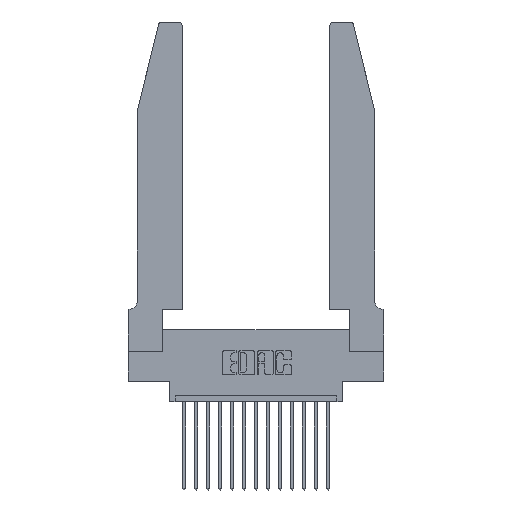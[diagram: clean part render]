
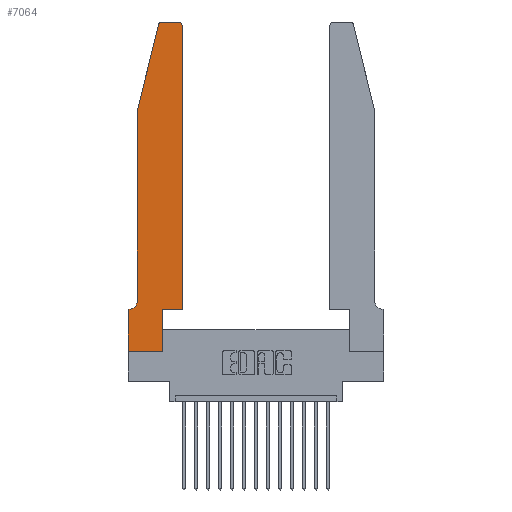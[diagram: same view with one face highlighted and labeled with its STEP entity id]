
A CAD part, top view. The second image highlights one B-rep face of the part: STEP entity #7064.
In plain terms, the highlighted planar face has unit normal (0, 0, 1).
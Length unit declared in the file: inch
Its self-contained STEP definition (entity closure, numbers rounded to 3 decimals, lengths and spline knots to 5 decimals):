
#534 = CARTESIAN_POINT ( 'NONE',  ( 0.2605, 2.75, 0.37 ) ) ;
#580 = ORIENTED_EDGE ( 'NONE', *, *, #16881, .T. ) ;
#1202 = FACE_OUTER_BOUND ( 'NONE', #14484, .T. ) ;
#1241 = VERTEX_POINT ( 'NONE', #10068 ) ;
#1324 = DIRECTION ( 'NONE',  ( 0., -1., 0. ) ) ;
#1689 = VECTOR ( 'NONE', #11862, 39.37008 ) ;
#1705 = LINE ( 'NONE', #17944, #4839 ) ;
#1820 = CARTESIAN_POINT ( 'NONE',  ( 0.0755, 0.42, 0.37 ) ) ;
#1891 = PLANE ( 'NONE',  #5517 ) ;
#2153 = CARTESIAN_POINT ( 'NONE',  ( 0.2865, 0.35, 0.37 ) ) ;
#2384 = ORIENTED_EDGE ( 'NONE', *, *, #9184, .T. ) ;
#2760 = DIRECTION ( 'NONE',  ( -0.239, -0.971, 0. ) ) ;
#2847 = ORIENTED_EDGE ( 'NONE', *, *, #17424, .T. ) ;
#3040 = LINE ( 'NONE', #8576, #8632 ) ;
#3177 = CARTESIAN_POINT ( 'NONE',  ( 0.284, 2.75, 0.37 ) ) ;
#3264 = ORIENTED_EDGE ( 'NONE', *, *, #9776, .T. ) ;
#3312 = DIRECTION ( 'NONE',  ( 0., 0., -1. ) ) ;
#3365 = VERTEX_POINT ( 'NONE', #1820 ) ;
#3503 = EDGE_CURVE ( 'NONE', #1241, #18596, #6241, .T. ) ;
#3515 = CIRCLE ( 'NONE', #6505, 0.03 ) ;
#3594 = CARTESIAN_POINT ( 'NONE',  ( 0.0755, 2., 0.37 ) ) ;
#3656 = LINE ( 'NONE', #2153, #18417 ) ;
#3830 = ORIENTED_EDGE ( 'NONE', *, *, #5843, .T. ) ;
#3967 = CARTESIAN_POINT ( 'NONE',  ( 0.4505, 0.35, 0.37 ) ) ;
#4839 = VECTOR ( 'NONE', #15191, 39.37008 ) ;
#5005 = ORIENTED_EDGE ( 'NONE', *, *, #8663, .T. ) ;
#5063 = CARTESIAN_POINT ( 'NONE',  ( 0.284, 2.72, 0.37 ) ) ;
#5140 = LINE ( 'NONE', #12147, #12791 ) ;
#5157 = CARTESIAN_POINT ( 'NONE',  ( 0.4505, 0.35, 0.37 ) ) ;
#5517 = AXIS2_PLACEMENT_3D ( 'NONE', #14723, #13571, #9292 ) ;
#5765 = CARTESIAN_POINT ( 'NONE',  ( 0.4205, 2.75, 0.37 ) ) ;
#5801 = ORIENTED_EDGE ( 'NONE', *, *, #14795, .T. ) ;
#5843 = EDGE_CURVE ( 'NONE', #7129, #14209, #3040, .T. ) ;
#5889 = AXIS2_PLACEMENT_3D ( 'NONE', #5063, #15081, #16521 ) ;
#6227 = VECTOR ( 'NONE', #12973, 39.37008 ) ;
#6241 = LINE ( 'NONE', #3967, #13441 ) ;
#6505 = AXIS2_PLACEMENT_3D ( 'NONE', #15580, #8442, #18453 ) ;
#6747 = CARTESIAN_POINT ( 'NONE',  ( 0.25487, 2.72718, 0.37 ) ) ;
#7064 = ADVANCED_FACE ( 'NONE', ( #1202 ), #1891, .T. ) ;
#7129 = VERTEX_POINT ( 'NONE', #6747 ) ;
#7432 = VERTEX_POINT ( 'NONE', #5765 ) ;
#7665 = VERTEX_POINT ( 'NONE', #8841 ) ;
#7791 = DIRECTION ( 'NONE',  ( 0., 1., 0. ) ) ;
#7884 = VECTOR ( 'NONE', #1324, 39.37008 ) ;
#8008 = VERTEX_POINT ( 'NONE', #9509 ) ;
#8344 = CARTESIAN_POINT ( 'NONE',  ( 0.4505, 2.72, 0.37 ) ) ;
#8442 = DIRECTION ( 'NONE',  ( 0., 0., 1. ) ) ;
#8545 = VECTOR ( 'NONE', #11761, 39.37008 ) ;
#8576 = CARTESIAN_POINT ( 'NONE',  ( 0.0755, 2., 0.37 ) ) ;
#8599 = ORIENTED_EDGE ( 'NONE', *, *, #11994, .T. ) ;
#8632 = VECTOR ( 'NONE', #2760, 39.37008 ) ;
#8640 = EDGE_CURVE ( 'NONE', #7665, #15462, #17827, .T. ) ;
#8663 = EDGE_CURVE ( 'NONE', #18596, #16634, #1705, .T. ) ;
#8713 = ORIENTED_EDGE ( 'NONE', *, *, #8640, .T. ) ;
#8841 = CARTESIAN_POINT ( 'NONE',  ( 0.0055, 0.35, 0.37 ) ) ;
#9184 = EDGE_CURVE ( 'NONE', #3365, #7665, #11392, .T. ) ;
#9233 = LINE ( 'NONE', #534, #8545 ) ;
#9292 = DIRECTION ( 'NONE',  ( 1., 0., 0. ) ) ;
#9509 = CARTESIAN_POINT ( 'NONE',  ( 0., 0., 0.37 ) ) ;
#9776 = EDGE_CURVE ( 'NONE', #16634, #7432, #3515, .T. ) ;
#9935 = CARTESIAN_POINT ( 'NONE',  ( 0., 0., 0.37 ) ) ;
#10060 = LINE ( 'NONE', #15683, #6227 ) ;
#10068 = CARTESIAN_POINT ( 'NONE',  ( 0.2865, 0.35, 0.37 ) ) ;
#10774 = VERTEX_POINT ( 'NONE', #11168 ) ;
#11168 = CARTESIAN_POINT ( 'NONE',  ( 0.2865, 0., 0.37 ) ) ;
#11321 = EDGE_CURVE ( 'NONE', #15462, #8008, #15965, .T. ) ;
#11392 = CIRCLE ( 'NONE', #16928, 0.07 ) ;
#11761 = DIRECTION ( 'NONE',  ( -1., 0., 0. ) ) ;
#11862 = DIRECTION ( 'NONE',  ( -1., 0., 0. ) ) ;
#11891 = VERTEX_POINT ( 'NONE', #3177 ) ;
#11919 = CARTESIAN_POINT ( 'NONE',  ( 0.0055, 0.42, 0.37 ) ) ;
#11994 = EDGE_CURVE ( 'NONE', #10774, #1241, #3656, .T. ) ;
#12083 = DIRECTION ( 'NONE',  ( 1., 0., 0. ) ) ;
#12147 = CARTESIAN_POINT ( 'NONE',  ( 0., 0., 0.37 ) ) ;
#12791 = VECTOR ( 'NONE', #12083, 39.37008 ) ;
#12973 = DIRECTION ( 'NONE',  ( 0., -1., 0. ) ) ;
#13344 = DIRECTION ( 'NONE',  ( -1., 0., 0. ) ) ;
#13441 = VECTOR ( 'NONE', #14167, 39.37008 ) ;
#13571 = DIRECTION ( 'NONE',  ( 0., 0., 1. ) ) ;
#14167 = DIRECTION ( 'NONE',  ( 1., 0., 0. ) ) ;
#14209 = VERTEX_POINT ( 'NONE', #3594 ) ;
#14484 = EDGE_LOOP ( 'NONE', ( #580, #2847, #3830, #5801, #2384, #8713, #16188, #16030, #8599, #15872, #5005, #3264 ) ) ;
#14723 = CARTESIAN_POINT ( 'NONE',  ( 0., 0.35, 0.37 ) ) ;
#14795 = EDGE_CURVE ( 'NONE', #14209, #3365, #10060, .T. ) ;
#15081 = DIRECTION ( 'NONE',  ( 0., 0., 1. ) ) ;
#15191 = DIRECTION ( 'NONE',  ( 0., 1., 0. ) ) ;
#15462 = VERTEX_POINT ( 'NONE', #16609 ) ;
#15580 = CARTESIAN_POINT ( 'NONE',  ( 0.4205, 2.72, 0.37 ) ) ;
#15683 = CARTESIAN_POINT ( 'NONE',  ( 0.0755, 2., 0.37 ) ) ;
#15872 = ORIENTED_EDGE ( 'NONE', *, *, #3503, .T. ) ;
#15965 = LINE ( 'NONE', #9935, #7884 ) ;
#16030 = ORIENTED_EDGE ( 'NONE', *, *, #17841, .T. ) ;
#16130 = CIRCLE ( 'NONE', #5889, 0.03 ) ;
#16131 = CARTESIAN_POINT ( 'NONE',  ( 0.0755, 0.35, 0.37 ) ) ;
#16188 = ORIENTED_EDGE ( 'NONE', *, *, #11321, .T. ) ;
#16521 = DIRECTION ( 'NONE',  ( 1., 0., 0. ) ) ;
#16609 = CARTESIAN_POINT ( 'NONE',  ( 0., 0.35, 0.37 ) ) ;
#16634 = VERTEX_POINT ( 'NONE', #8344 ) ;
#16881 = EDGE_CURVE ( 'NONE', #7432, #11891, #9233, .T. ) ;
#16928 = AXIS2_PLACEMENT_3D ( 'NONE', #11919, #3312, #13344 ) ;
#17424 = EDGE_CURVE ( 'NONE', #11891, #7129, #16130, .T. ) ;
#17827 = LINE ( 'NONE', #16131, #1689 ) ;
#17841 = EDGE_CURVE ( 'NONE', #8008, #10774, #5140, .T. ) ;
#17944 = CARTESIAN_POINT ( 'NONE',  ( 0.4505, 0.35, 0.37 ) ) ;
#18417 = VECTOR ( 'NONE', #7791, 39.37008 ) ;
#18453 = DIRECTION ( 'NONE',  ( 1., 0., 0. ) ) ;
#18596 = VERTEX_POINT ( 'NONE', #5157 ) ;
